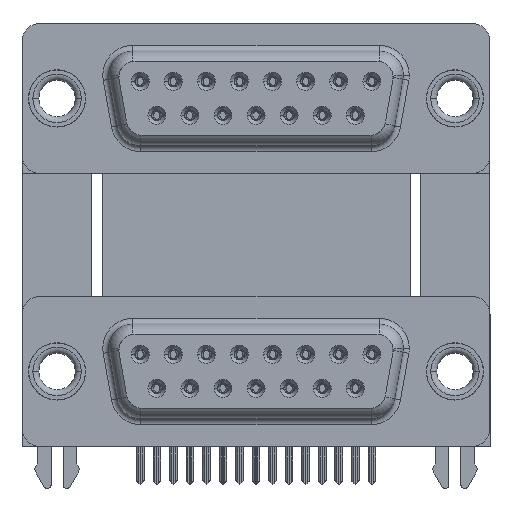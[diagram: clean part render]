
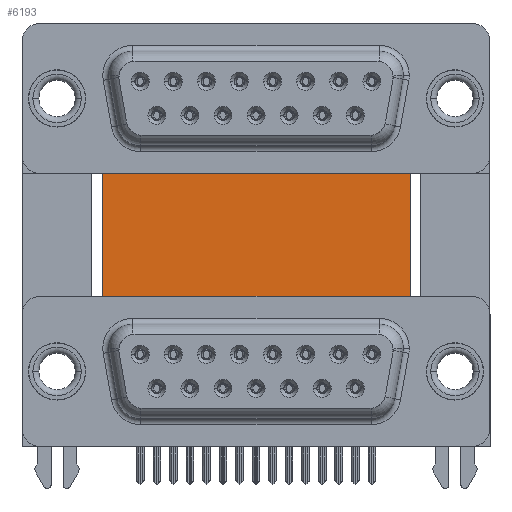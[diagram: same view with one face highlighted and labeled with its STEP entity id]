
A CAD part, top view. The second image highlights one B-rep face of the part: STEP entity #6193.
In plain terms, the highlighted planar face has unit normal (0, 0, 1).
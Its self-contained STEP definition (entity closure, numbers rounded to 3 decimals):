
#292 = VECTOR ( 'NONE', #18292, 1000. ) ;
#2153 = LINE ( 'NONE', #42440, #14418 ) ;
#4354 = CARTESIAN_POINT ( 'NONE',  ( 3.79, -3.735, -12. ) ) ;
#5099 = VERTEX_POINT ( 'NONE', #43762 ) ;
#5983 = VERTEX_POINT ( 'NONE', #19634 ) ;
#6193 = ADVANCED_FACE ( 'NONE', ( #14711 ), #40352, .F. ) ;
#7815 = CARTESIAN_POINT ( 'NONE',  ( 3.79, 16.585, -12. ) ) ;
#7958 = ORIENTED_EDGE ( 'NONE', *, *, #31593, .F. ) ;
#11279 = DIRECTION ( 'NONE',  ( 0., 0., -1. ) ) ;
#11877 = EDGE_CURVE ( 'NONE', #5983, #27459, #30483, .T. ) ;
#12301 = ORIENTED_EDGE ( 'NONE', *, *, #11877, .T. ) ;
#14418 = VECTOR ( 'NONE', #31924, 1000. ) ;
#14711 = FACE_OUTER_BOUND ( 'NONE', #18811, .T. ) ;
#15321 = EDGE_CURVE ( 'NONE', #35149, #5099, #2153, .T. ) ;
#15578 = DIRECTION ( 'NONE',  ( 1., 0., 0. ) ) ;
#18292 = DIRECTION ( 'NONE',  ( 0., -1., 0. ) ) ;
#18352 = DIRECTION ( 'NONE',  ( -1., 0., 0. ) ) ;
#18811 = EDGE_LOOP ( 'NONE', ( #34297, #23600, #7958, #12301 ) ) ;
#19634 = CARTESIAN_POINT ( 'NONE',  ( 3.79, 16.585, -12. ) ) ;
#21875 = LINE ( 'NONE', #41153, #43414 ) ;
#22872 = LINE ( 'NONE', #4354, #33487 ) ;
#23600 = ORIENTED_EDGE ( 'NONE', *, *, #15321, .F. ) ;
#26869 = CARTESIAN_POINT ( 'NONE',  ( 29.58, 16.585, -12. ) ) ;
#27459 = VERTEX_POINT ( 'NONE', #44159 ) ;
#30483 = LINE ( 'NONE', #7815, #292 ) ;
#31593 = EDGE_CURVE ( 'NONE', #5983, #35149, #21875, .T. ) ;
#31924 = DIRECTION ( 'NONE',  ( 0., -1., 0. ) ) ;
#33487 = VECTOR ( 'NONE', #15578, 1000. ) ;
#34297 = ORIENTED_EDGE ( 'NONE', *, *, #37031, .T. ) ;
#34431 = AXIS2_PLACEMENT_3D ( 'NONE', #37153, #11279, #18352 ) ;
#35149 = VERTEX_POINT ( 'NONE', #26869 ) ;
#37031 = EDGE_CURVE ( 'NONE', #27459, #5099, #22872, .T. ) ;
#37153 = CARTESIAN_POINT ( 'NONE',  ( 3.79, 16.585, -12. ) ) ;
#40352 = PLANE ( 'NONE',  #34431 ) ;
#41153 = CARTESIAN_POINT ( 'NONE',  ( 3.79, 16.585, -12. ) ) ;
#42440 = CARTESIAN_POINT ( 'NONE',  ( 29.58, 16.585, -12. ) ) ;
#43414 = VECTOR ( 'NONE', #48274, 1000. ) ;
#43762 = CARTESIAN_POINT ( 'NONE',  ( 29.58, -3.735, -12. ) ) ;
#44159 = CARTESIAN_POINT ( 'NONE',  ( 3.79, -3.735, -12. ) ) ;
#48274 = DIRECTION ( 'NONE',  ( 1., 0., 0. ) ) ;
